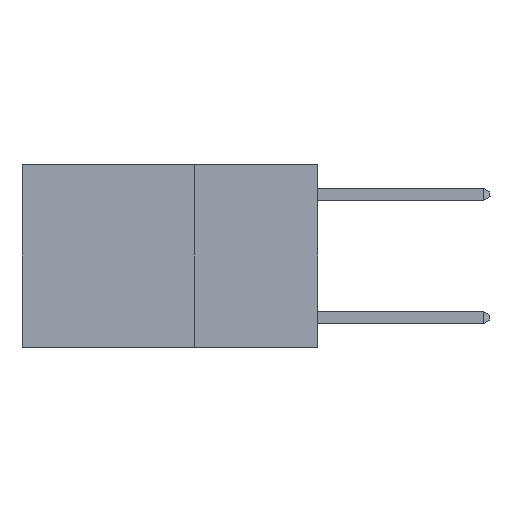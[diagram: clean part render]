
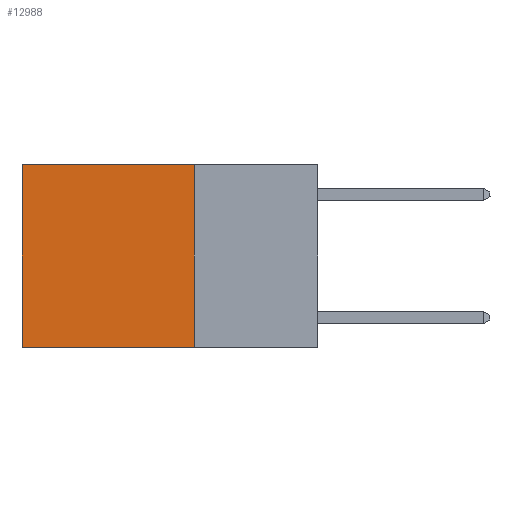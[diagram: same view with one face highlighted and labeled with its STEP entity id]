
A CAD part, left-side view. The second image highlights one B-rep face of the part: STEP entity #12988.
In plain terms, the highlighted planar face has unit normal (-1, 0, 0).
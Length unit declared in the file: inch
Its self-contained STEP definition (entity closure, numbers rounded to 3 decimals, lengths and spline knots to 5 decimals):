
#389 = VERTEX_POINT ( 'NONE', #18941 ) ;
#783 = EDGE_CURVE ( 'NONE', #14821, #389, #4458, .T. ) ;
#1359 = EDGE_CURVE ( 'NONE', #7418, #18925, #19639, .T. ) ;
#1623 = VECTOR ( 'NONE', #11562, 39.37008 ) ;
#2774 = CARTESIAN_POINT ( 'NONE',  ( 0.2625, 0.25, 0. ) ) ;
#2967 = DIRECTION ( 'NONE',  ( 0., 0., -1. ) ) ;
#3045 = PLANE ( 'NONE',  #14061 ) ;
#3253 = CARTESIAN_POINT ( 'NONE',  ( 0.2625, 0.25, -0.37 ) ) ;
#3509 = VECTOR ( 'NONE', #16097, 39.37008 ) ;
#4458 = LINE ( 'NONE', #9441, #3509 ) ;
#5922 = ORIENTED_EDGE ( 'NONE', *, *, #13974, .T. ) ;
#6277 = ORIENTED_EDGE ( 'NONE', *, *, #1359, .F. ) ;
#6714 = ORIENTED_EDGE ( 'NONE', *, *, #8319, .F. ) ;
#6965 = VECTOR ( 'NONE', #2967, 39.37008 ) ;
#7418 = VERTEX_POINT ( 'NONE', #2774 ) ;
#7571 = DIRECTION ( 'NONE',  ( 0., 1., 0. ) ) ;
#8319 = EDGE_CURVE ( 'NONE', #18925, #389, #9224, .T. ) ;
#9224 = LINE ( 'NONE', #13925, #15297 ) ;
#9441 = CARTESIAN_POINT ( 'NONE',  ( 0.2625, 0.6, 0. ) ) ;
#9804 = CARTESIAN_POINT ( 'NONE',  ( 0.2625, 0.25, 0. ) ) ;
#11301 = CARTESIAN_POINT ( 'NONE',  ( 0.2625, 0.6, 0. ) ) ;
#11357 = CARTESIAN_POINT ( 'NONE',  ( 0.2625, 0.25, 0. ) ) ;
#11562 = DIRECTION ( 'NONE',  ( 0., 1., 0. ) ) ;
#12600 = EDGE_LOOP ( 'NONE', ( #16634, #6714, #6277, #5922 ) ) ;
#12988 = ADVANCED_FACE ( 'NONE', ( #19823 ), #3045, .F. ) ;
#13076 = DIRECTION ( 'NONE',  ( 1., 0., 0. ) ) ;
#13925 = CARTESIAN_POINT ( 'NONE',  ( 0.2625, 0.25, -0.37 ) ) ;
#13974 = EDGE_CURVE ( 'NONE', #7418, #14821, #17936, .T. ) ;
#14061 = AXIS2_PLACEMENT_3D ( 'NONE', #18007, #13076, #17802 ) ;
#14821 = VERTEX_POINT ( 'NONE', #11301 ) ;
#15297 = VECTOR ( 'NONE', #7571, 39.37008 ) ;
#16097 = DIRECTION ( 'NONE',  ( 0., 0., -1. ) ) ;
#16634 = ORIENTED_EDGE ( 'NONE', *, *, #783, .T. ) ;
#17802 = DIRECTION ( 'NONE',  ( 0., 0., -1. ) ) ;
#17936 = LINE ( 'NONE', #9804, #1623 ) ;
#18007 = CARTESIAN_POINT ( 'NONE',  ( 0.2625, 0.25, 0. ) ) ;
#18925 = VERTEX_POINT ( 'NONE', #3253 ) ;
#18941 = CARTESIAN_POINT ( 'NONE',  ( 0.2625, 0.6, -0.37 ) ) ;
#19639 = LINE ( 'NONE', #11357, #6965 ) ;
#19823 = FACE_OUTER_BOUND ( 'NONE', #12600, .T. ) ;
